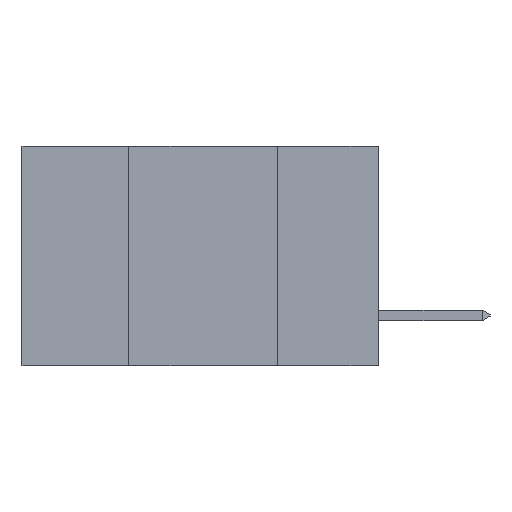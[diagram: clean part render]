
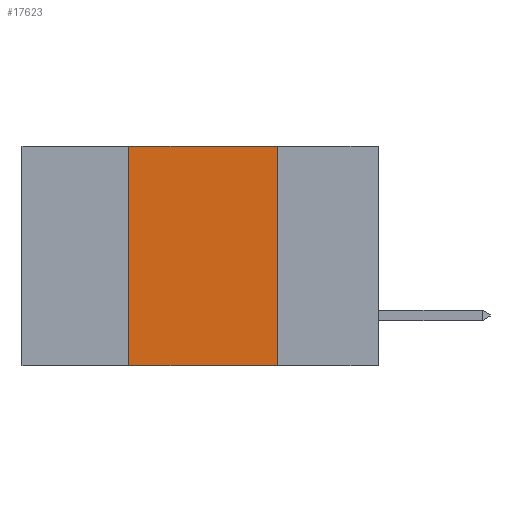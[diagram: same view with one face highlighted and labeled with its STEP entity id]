
A CAD part, left-side view. The second image highlights one B-rep face of the part: STEP entity #17623.
In plain terms, the highlighted planar face has unit normal (-1, 0, 0).
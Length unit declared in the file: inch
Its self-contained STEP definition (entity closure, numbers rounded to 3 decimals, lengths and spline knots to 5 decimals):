
#79 = VECTOR ( 'NONE', #5219, 39.37008 ) ;
#909 = ORIENTED_EDGE ( 'NONE', *, *, #15824, .F. ) ;
#1933 = VERTEX_POINT ( 'NONE', #11582 ) ;
#2678 = PLANE ( 'NONE',  #18306 ) ;
#3111 = VERTEX_POINT ( 'NONE', #13292 ) ;
#4257 = LINE ( 'NONE', #12922, #79 ) ;
#4697 = VERTEX_POINT ( 'NONE', #17803 ) ;
#5219 = DIRECTION ( 'NONE',  ( 0., 0., -1. ) ) ;
#5729 = EDGE_LOOP ( 'NONE', ( #909, #12550, #17082, #7755 ) ) ;
#5796 = DIRECTION ( 'NONE',  ( 0., 0., -1. ) ) ;
#6371 = CARTESIAN_POINT ( 'NONE',  ( 0., 0.6, -0.37 ) ) ;
#6438 = DIRECTION ( 'NONE',  ( 0., -1., 0. ) ) ;
#6493 = VECTOR ( 'NONE', #6438, 39.37008 ) ;
#6958 = EDGE_CURVE ( 'NONE', #8721, #4697, #10606, .T. ) ;
#7755 = ORIENTED_EDGE ( 'NONE', *, *, #6958, .T. ) ;
#8721 = VERTEX_POINT ( 'NONE', #9913 ) ;
#9014 = CARTESIAN_POINT ( 'NONE',  ( 0., 0.6, 0. ) ) ;
#9913 = CARTESIAN_POINT ( 'NONE',  ( 0., 0.42, -0.37 ) ) ;
#10015 = VECTOR ( 'NONE', #16331, 39.37008 ) ;
#10257 = CARTESIAN_POINT ( 'NONE',  ( 0., 0.42, -0.37 ) ) ;
#10283 = VECTOR ( 'NONE', #10529, 39.37008 ) ;
#10529 = DIRECTION ( 'NONE',  ( 0., -1., 0. ) ) ;
#10606 = LINE ( 'NONE', #6371, #6493 ) ;
#10936 = LINE ( 'NONE', #10257, #10015 ) ;
#11582 = CARTESIAN_POINT ( 'NONE',  ( 0., 0.17, 0. ) ) ;
#11698 = EDGE_CURVE ( 'NONE', #3111, #1933, #13872, .T. ) ;
#12550 = ORIENTED_EDGE ( 'NONE', *, *, #11698, .F. ) ;
#12922 = CARTESIAN_POINT ( 'NONE',  ( 0., 0.17, -0.37 ) ) ;
#13292 = CARTESIAN_POINT ( 'NONE',  ( 0., 0.42, 0. ) ) ;
#13499 = CARTESIAN_POINT ( 'NONE',  ( 0., 0.6, 0. ) ) ;
#13597 = FACE_OUTER_BOUND ( 'NONE', #5729, .T. ) ;
#13872 = LINE ( 'NONE', #9014, #10283 ) ;
#15027 = DIRECTION ( 'NONE',  ( 1., 0., 0. ) ) ;
#15824 = EDGE_CURVE ( 'NONE', #1933, #4697, #4257, .T. ) ;
#16331 = DIRECTION ( 'NONE',  ( 0., 0., 1. ) ) ;
#17082 = ORIENTED_EDGE ( 'NONE', *, *, #18195, .F. ) ;
#17623 = ADVANCED_FACE ( 'NONE', ( #13597 ), #2678, .F. ) ;
#17803 = CARTESIAN_POINT ( 'NONE',  ( 0., 0.17, -0.37 ) ) ;
#18195 = EDGE_CURVE ( 'NONE', #8721, #3111, #10936, .T. ) ;
#18306 = AXIS2_PLACEMENT_3D ( 'NONE', #13499, #15027, #5796 ) ;
